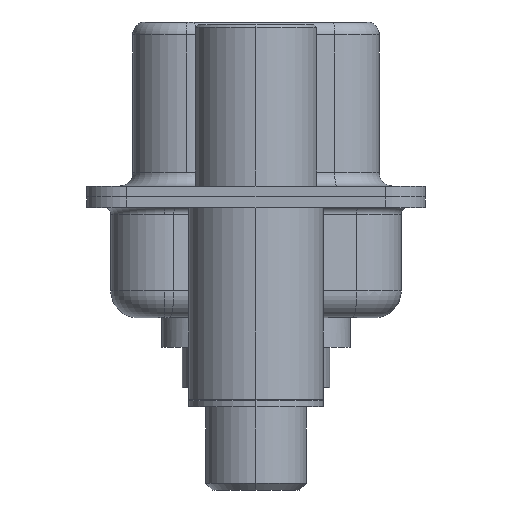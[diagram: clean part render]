
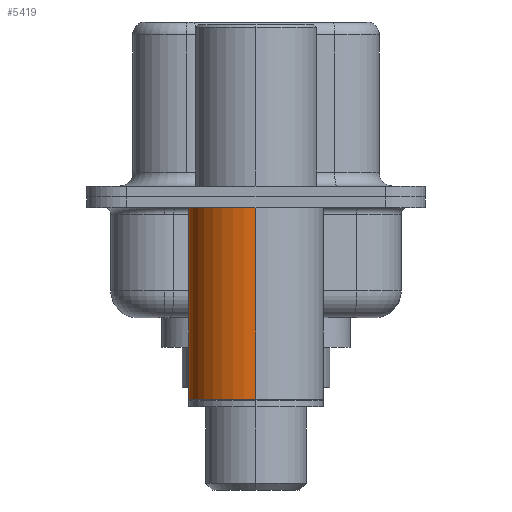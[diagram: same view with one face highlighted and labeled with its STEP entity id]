
A CAD part, left-side view. The second image highlights one B-rep face of the part: STEP entity #5419.
In plain terms, the highlighted cylindrical face has radius 2.5 mm (diameter 5 mm), a partial arc.
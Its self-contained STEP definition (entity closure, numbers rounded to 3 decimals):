
#166 = DIRECTION ( 'NONE',  ( 0., 0., 1. ) ) ;
#975 = DIRECTION ( 'NONE',  ( 1., 0., 0. ) ) ;
#1503 = VERTEX_POINT ( 'NONE', #7832 ) ;
#1600 = VERTEX_POINT ( 'NONE', #15902 ) ;
#1765 = CARTESIAN_POINT ( 'NONE',  ( -2.5, 0., -7.525 ) ) ;
#2077 = VERTEX_POINT ( 'NONE', #1765 ) ;
#2397 = CIRCLE ( 'NONE', #4475, 2.5 ) ;
#2434 = EDGE_CURVE ( 'NONE', #1503, #1600, #2766, .T. ) ;
#2442 = ORIENTED_EDGE ( 'NONE', *, *, #14171, .T. ) ;
#2612 = ORIENTED_EDGE ( 'NONE', *, *, #9826, .F. ) ;
#2745 = LINE ( 'NONE', #12764, #6430 ) ;
#2766 = LINE ( 'NONE', #8054, #13112 ) ;
#3027 = CARTESIAN_POINT ( 'NONE',  ( 0., 0., 0.581 ) ) ;
#3177 = ORIENTED_EDGE ( 'NONE', *, *, #2434, .F. ) ;
#4475 = AXIS2_PLACEMENT_3D ( 'NONE', #17067, #9261, #975 ) ;
#4551 = DIRECTION ( 'NONE',  ( 0., 0., 1. ) ) ;
#4639 = CARTESIAN_POINT ( 'NONE',  ( -2.5, 0., -0.4 ) ) ;
#4673 = FACE_OUTER_BOUND ( 'NONE', #15472, .T. ) ;
#4957 = VERTEX_POINT ( 'NONE', #4639 ) ;
#5046 = CIRCLE ( 'NONE', #11684, 2.5 ) ;
#5362 = AXIS2_PLACEMENT_3D ( 'NONE', #3027, #166, #16316 ) ;
#5419 = ADVANCED_FACE ( 'NONE', ( #4673 ), #14832, .T. ) ;
#6430 = VECTOR ( 'NONE', #14038, 1000. ) ;
#6651 = DIRECTION ( 'NONE',  ( 0., 0., 1. ) ) ;
#7832 = CARTESIAN_POINT ( 'NONE',  ( 2.5, 0., -7.525 ) ) ;
#8054 = CARTESIAN_POINT ( 'NONE',  ( 2.5, 0., 0.581 ) ) ;
#9261 = DIRECTION ( 'NONE',  ( 0., 0., 1. ) ) ;
#9826 = EDGE_CURVE ( 'NONE', #1600, #4957, #2397, .T. ) ;
#11684 = AXIS2_PLACEMENT_3D ( 'NONE', #12617, #4551, #13883 ) ;
#12617 = CARTESIAN_POINT ( 'NONE',  ( 0., 0., -7.525 ) ) ;
#12764 = CARTESIAN_POINT ( 'NONE',  ( -2.5, 0., 0.581 ) ) ;
#13112 = VECTOR ( 'NONE', #6651, 1000. ) ;
#13883 = DIRECTION ( 'NONE',  ( 1., 0., 0. ) ) ;
#14038 = DIRECTION ( 'NONE',  ( 0., 0., 1. ) ) ;
#14171 = EDGE_CURVE ( 'NONE', #2077, #4957, #2745, .T. ) ;
#14343 = ORIENTED_EDGE ( 'NONE', *, *, #15031, .T. ) ;
#14832 = CYLINDRICAL_SURFACE ( 'NONE', #5362, 2.5 ) ;
#15031 = EDGE_CURVE ( 'NONE', #1503, #2077, #5046, .T. ) ;
#15472 = EDGE_LOOP ( 'NONE', ( #14343, #2442, #2612, #3177 ) ) ;
#15902 = CARTESIAN_POINT ( 'NONE',  ( 2.5, 0., -0.4 ) ) ;
#16316 = DIRECTION ( 'NONE',  ( 1., 0., 0. ) ) ;
#17067 = CARTESIAN_POINT ( 'NONE',  ( 0., 0., -0.4 ) ) ;
